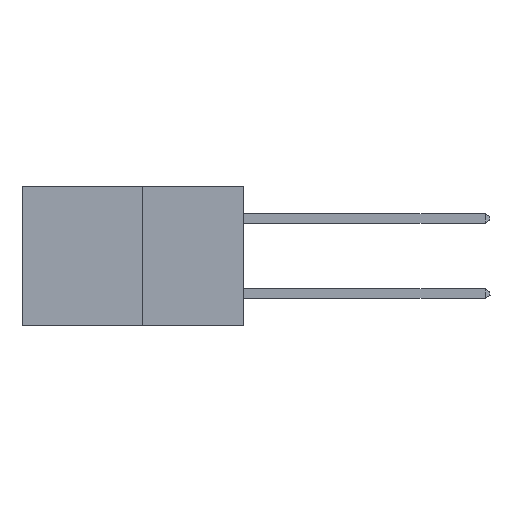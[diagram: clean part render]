
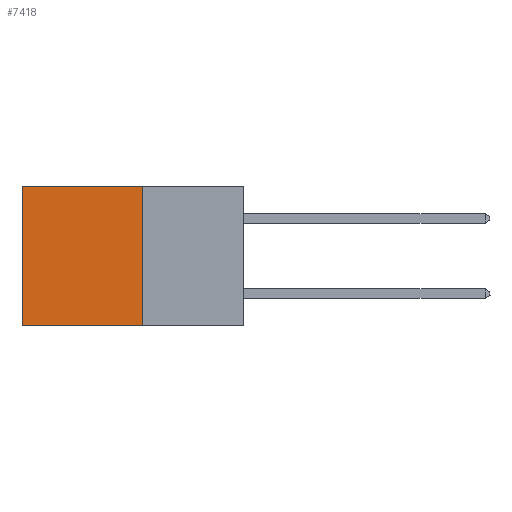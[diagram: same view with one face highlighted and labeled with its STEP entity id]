
A CAD part, left-side view. The second image highlights one B-rep face of the part: STEP entity #7418.
In plain terms, the highlighted planar face has unit normal (-1, 0, 0).
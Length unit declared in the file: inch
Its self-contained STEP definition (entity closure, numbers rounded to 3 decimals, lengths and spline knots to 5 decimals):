
#4 = LINE ( 'NONE', #9845, #20828 ) ;
#54 = DIRECTION ( 'NONE',  ( 0., 0., -1. ) ) ;
#96 = EDGE_CURVE ( 'NONE', #2469, #5108, #271, .T. ) ;
#271 = LINE ( 'NONE', #20973, #8492 ) ;
#985 = VERTEX_POINT ( 'NONE', #13187 ) ;
#2008 = DIRECTION ( 'NONE',  ( 0., 0., -1. ) ) ;
#2084 = ORIENTED_EDGE ( 'NONE', *, *, #10778, .T. ) ;
#2258 = CARTESIAN_POINT ( 'NONE',  ( 0.277, 0.59, -0.37 ) ) ;
#2469 = VERTEX_POINT ( 'NONE', #18222 ) ;
#3167 = AXIS2_PLACEMENT_3D ( 'NONE', #7215, #6796, #54 ) ;
#3451 = ORIENTED_EDGE ( 'NONE', *, *, #96, .F. ) ;
#4928 = EDGE_CURVE ( 'NONE', #2469, #5822, #4, .T. ) ;
#5108 = VERTEX_POINT ( 'NONE', #14511 ) ;
#5822 = VERTEX_POINT ( 'NONE', #11503 ) ;
#6186 = DIRECTION ( 'NONE',  ( 0., 1., 0. ) ) ;
#6311 = EDGE_LOOP ( 'NONE', ( #2084, #9536, #3451, #9983 ) ) ;
#6796 = DIRECTION ( 'NONE',  ( 1., 0., 0. ) ) ;
#7215 = CARTESIAN_POINT ( 'NONE',  ( 0.277, 0.27, -0.37 ) ) ;
#7329 = CARTESIAN_POINT ( 'NONE',  ( 0.277, 0.27, -0.37 ) ) ;
#7418 = ADVANCED_FACE ( 'NONE', ( #8359 ), #12554, .F. ) ;
#7719 = DIRECTION ( 'NONE',  ( 0., 0., -1. ) ) ;
#7976 = VECTOR ( 'NONE', #12308, 39.37008 ) ;
#8359 = FACE_OUTER_BOUND ( 'NONE', #6311, .T. ) ;
#8492 = VECTOR ( 'NONE', #7719, 39.37008 ) ;
#9536 = ORIENTED_EDGE ( 'NONE', *, *, #12750, .F. ) ;
#9845 = CARTESIAN_POINT ( 'NONE',  ( 0.277, 0.27, 0. ) ) ;
#9983 = ORIENTED_EDGE ( 'NONE', *, *, #4928, .T. ) ;
#10778 = EDGE_CURVE ( 'NONE', #5822, #985, #15060, .T. ) ;
#11503 = CARTESIAN_POINT ( 'NONE',  ( 0.277, 0.59, 0. ) ) ;
#12308 = DIRECTION ( 'NONE',  ( 0., 1., 0. ) ) ;
#12554 = PLANE ( 'NONE',  #3167 ) ;
#12750 = EDGE_CURVE ( 'NONE', #5108, #985, #21120, .T. ) ;
#13187 = CARTESIAN_POINT ( 'NONE',  ( 0.277, 0.59, -0.37 ) ) ;
#14511 = CARTESIAN_POINT ( 'NONE',  ( 0.277, 0.27, -0.37 ) ) ;
#15060 = LINE ( 'NONE', #2258, #18420 ) ;
#18222 = CARTESIAN_POINT ( 'NONE',  ( 0.277, 0.27, 0. ) ) ;
#18420 = VECTOR ( 'NONE', #2008, 39.37008 ) ;
#20828 = VECTOR ( 'NONE', #6186, 39.37008 ) ;
#20973 = CARTESIAN_POINT ( 'NONE',  ( 0.277, 0.27, -0.37 ) ) ;
#21120 = LINE ( 'NONE', #7329, #7976 ) ;
